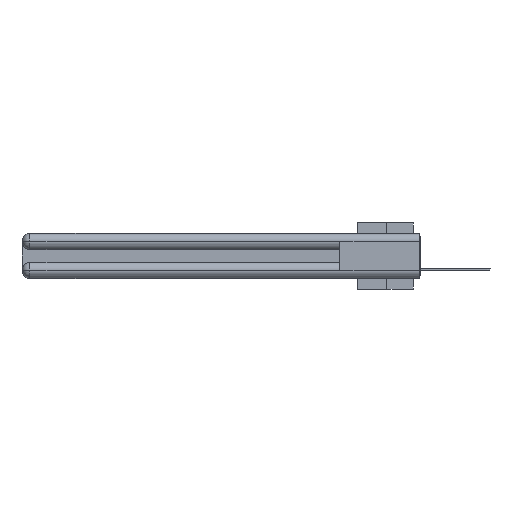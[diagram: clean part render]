
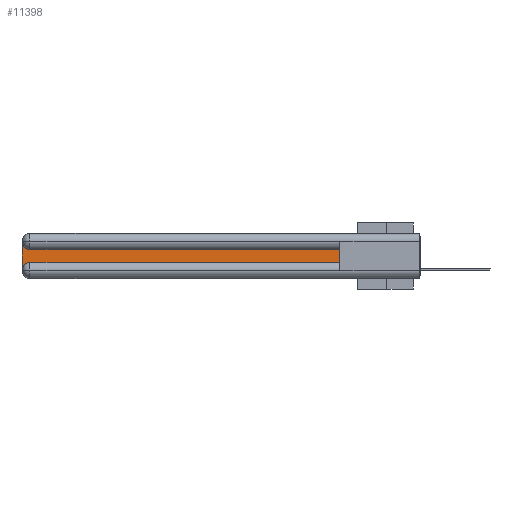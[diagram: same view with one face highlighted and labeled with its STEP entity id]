
A CAD part, left-side view. The second image highlights one B-rep face of the part: STEP entity #11398.
In plain terms, the highlighted planar face has unit normal (-1, 0, 0).
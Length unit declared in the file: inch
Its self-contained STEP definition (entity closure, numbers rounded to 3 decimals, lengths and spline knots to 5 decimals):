
#1924 = AXIS2_PLACEMENT_3D ( 'NONE', #9768, #31275, #3493 ) ;
#2688 = VECTOR ( 'NONE', #21066, 39.37008 ) ;
#3493 = DIRECTION ( 'NONE',  ( 0., 0., -1. ) ) ;
#4796 = EDGE_CURVE ( 'NONE', #21875, #5248, #17452, .T. ) ;
#4858 = EDGE_CURVE ( 'NONE', #22771, #7561, #14225, .T. ) ;
#5248 = VERTEX_POINT ( 'NONE', #33882 ) ;
#5782 = VECTOR ( 'NONE', #30237, 39.37008 ) ;
#6355 = EDGE_CURVE ( 'NONE', #30762, #17312, #39762, .T. ) ;
#7460 = EDGE_CURVE ( 'NONE', #5248, #22771, #37992, .T. ) ;
#7561 = VERTEX_POINT ( 'NONE', #26215 ) ;
#8164 = PLANE ( 'NONE',  #32649 ) ;
#9768 = CARTESIAN_POINT ( 'NONE',  ( 0.075, 2.94, -0.2775 ) ) ;
#9994 = CARTESIAN_POINT ( 'NONE',  ( 0.075, 3., -0.2175 ) ) ;
#11192 = CARTESIAN_POINT ( 'NONE',  ( 0.075, 0.6, -0.2175 ) ) ;
#11398 = ADVANCED_FACE ( 'NONE', ( #23547 ), #8164, .F. ) ;
#11796 = EDGE_CURVE ( 'NONE', #17312, #21875, #14594, .T. ) ;
#14225 = CIRCLE ( 'NONE', #1924, 0.06 ) ;
#14256 = CARTESIAN_POINT ( 'NONE',  ( 0.075, 2.94, -0.0625 ) ) ;
#14594 = LINE ( 'NONE', #24115, #2688 ) ;
#16041 = DIRECTION ( 'NONE',  ( 0., 0., -1. ) ) ;
#17068 = CARTESIAN_POINT ( 'NONE',  ( 0.075, 2.94, -0.1225 ) ) ;
#17312 = VERTEX_POINT ( 'NONE', #35119 ) ;
#17452 = CIRCLE ( 'NONE', #29139, 0.06 ) ;
#18682 = VECTOR ( 'NONE', #22332, 39.37008 ) ;
#18872 = EDGE_CURVE ( 'NONE', #7561, #30762, #39154, .T. ) ;
#21066 = DIRECTION ( 'NONE',  ( 0., 1., 0. ) ) ;
#21875 = VERTEX_POINT ( 'NONE', #17068 ) ;
#22073 = ORIENTED_EDGE ( 'NONE', *, *, #4858, .T. ) ;
#22332 = DIRECTION ( 'NONE',  ( 0., 0., -1. ) ) ;
#22771 = VERTEX_POINT ( 'NONE', #38159 ) ;
#23547 = FACE_OUTER_BOUND ( 'NONE', #32880, .T. ) ;
#24115 = CARTESIAN_POINT ( 'NONE',  ( 0.075, 0.6, -0.1225 ) ) ;
#24127 = CARTESIAN_POINT ( 'NONE',  ( 0.075, 0.6, -0.2175 ) ) ;
#26215 = CARTESIAN_POINT ( 'NONE',  ( 0.075, 2.94, -0.2175 ) ) ;
#26268 = VECTOR ( 'NONE', #27403, 39.37008 ) ;
#26678 = ORIENTED_EDGE ( 'NONE', *, *, #11796, .T. ) ;
#27037 = DIRECTION ( 'NONE',  ( 0., 0., -1. ) ) ;
#27403 = DIRECTION ( 'NONE',  ( 0., 0., 1. ) ) ;
#28627 = CARTESIAN_POINT ( 'NONE',  ( 0.075, 3., -0.1225 ) ) ;
#29139 = AXIS2_PLACEMENT_3D ( 'NONE', #14256, #39009, #27037 ) ;
#30173 = ORIENTED_EDGE ( 'NONE', *, *, #18872, .T. ) ;
#30237 = DIRECTION ( 'NONE',  ( 0., -1., 0. ) ) ;
#30762 = VERTEX_POINT ( 'NONE', #35190 ) ;
#30968 = ORIENTED_EDGE ( 'NONE', *, *, #6355, .T. ) ;
#31275 = DIRECTION ( 'NONE',  ( 1., 0., 0. ) ) ;
#32649 = AXIS2_PLACEMENT_3D ( 'NONE', #28627, #37741, #16041 ) ;
#32744 = ORIENTED_EDGE ( 'NONE', *, *, #7460, .T. ) ;
#32880 = EDGE_LOOP ( 'NONE', ( #26678, #38697, #32744, #22073, #30173, #30968 ) ) ;
#33882 = CARTESIAN_POINT ( 'NONE',  ( 0.075, 3., -0.0625 ) ) ;
#35119 = CARTESIAN_POINT ( 'NONE',  ( 0.075, 0.6, -0.1225 ) ) ;
#35190 = CARTESIAN_POINT ( 'NONE',  ( 0.075, 0.6, -0.2175 ) ) ;
#37741 = DIRECTION ( 'NONE',  ( 1., 0., 0. ) ) ;
#37992 = LINE ( 'NONE', #9994, #18682 ) ;
#38159 = CARTESIAN_POINT ( 'NONE',  ( 0.075, 3., -0.2775 ) ) ;
#38697 = ORIENTED_EDGE ( 'NONE', *, *, #4796, .T. ) ;
#39009 = DIRECTION ( 'NONE',  ( 1., 0., 0. ) ) ;
#39154 = LINE ( 'NONE', #24127, #5782 ) ;
#39762 = LINE ( 'NONE', #11192, #26268 ) ;
